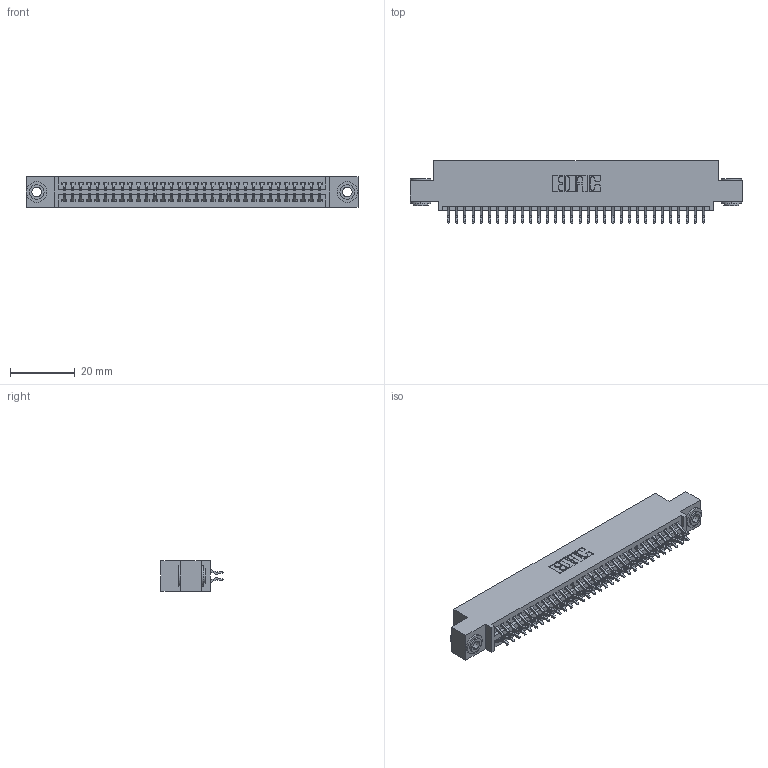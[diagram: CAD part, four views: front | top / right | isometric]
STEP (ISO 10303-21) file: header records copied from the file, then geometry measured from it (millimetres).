
FILE_DESCRIPTION (( 'STEP AP203' ), '1' );
FILE_NAME ('345-064-556-503.STEP', '2018-09-28T09:30:23', ( '' ), ( '' ), 'SwSTEP 2.0', 'SolidWorks 2016', '' );
FILE_SCHEMA (( 'CONFIG_CONTROL_DESIGN' ));
Length unit declared in the file: inch
Products named in the file (4): 345-064-556-503; 345-292-001_556 Tail; 345-250-002_345-250-002-102; 345 Part_0.110 Offset - 0.156 Dia-TH
Assembly tree (67 placements, depth 2):
  345-064-556-503
    345 Part_0.110 Offset - 0.156 Dia-TH
    345-292-001_556 Tail  x64
    345-250-002_345-250-002-102  x2
Bounding box: 102.49 x 19.24 x 9.4 mm (x, y, z)
Volume: 9806.6 mm3; surface area: 14543.8 mm2
Topology: 67 solids, 67 shells, 3752 faces, 11117 edges, 7322 vertices
Faces by surface type: plane 2462, cylinder 1282, cone 8
Entity records: 27456 total; most frequent: CARTESIAN_POINT 4603, ORIENTED_EDGE 4518, DIRECTION 4089, EDGE_CURVE 2259, VECTOR 1967, LINE 1967, VERTEX_POINT 1502, AXIS2_PLACEMENT_3D 1061
